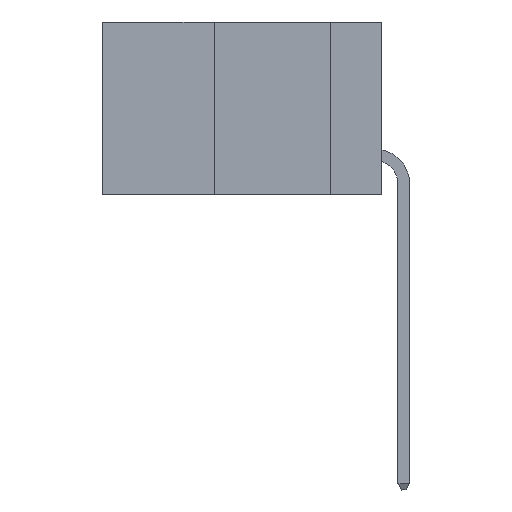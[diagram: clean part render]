
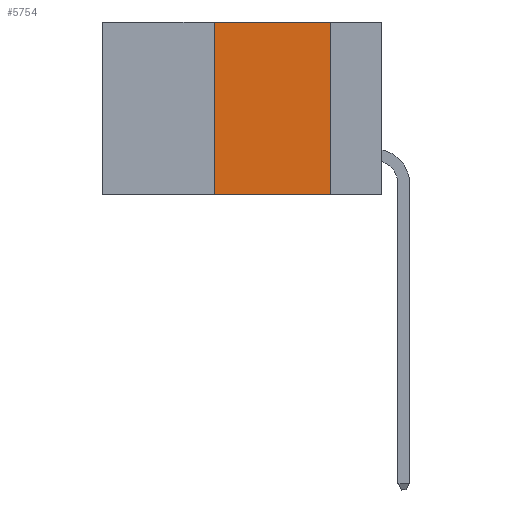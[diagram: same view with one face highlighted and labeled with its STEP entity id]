
A CAD part, left-side view. The second image highlights one B-rep face of the part: STEP entity #5754.
In plain terms, the highlighted planar face has unit normal (-1, 0, 0).
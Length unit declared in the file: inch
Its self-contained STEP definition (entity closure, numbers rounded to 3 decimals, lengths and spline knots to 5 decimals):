
#187 = DIRECTION ( 'NONE',  ( 0., -1., 0. ) ) ;
#1971 = EDGE_CURVE ( 'NONE', #26377, #19439, #18614, .T. ) ;
#2101 = VECTOR ( 'NONE', #187, 39.37008 ) ;
#5494 = EDGE_CURVE ( 'NONE', #26377, #20119, #9552, .T. ) ;
#5586 = CARTESIAN_POINT ( 'NONE',  ( 0., 0.6, 0. ) ) ;
#5754 = ADVANCED_FACE ( 'NONE', ( #17334 ), #20663, .F. ) ;
#5991 = VECTOR ( 'NONE', #29665, 39.37008 ) ;
#6948 = DIRECTION ( 'NONE',  ( 0., 0., -1. ) ) ;
#7227 = VECTOR ( 'NONE', #6948, 39.37008 ) ;
#7928 = CARTESIAN_POINT ( 'NONE',  ( 0., 0.6, 0. ) ) ;
#8650 = EDGE_LOOP ( 'NONE', ( #11639, #40400, #13855, #16289 ) ) ;
#9552 = LINE ( 'NONE', #42589, #5991 ) ;
#10237 = CARTESIAN_POINT ( 'NONE',  ( 0., 0.6, -0.37 ) ) ;
#11639 = ORIENTED_EDGE ( 'NONE', *, *, #19722, .F. ) ;
#13381 = LINE ( 'NONE', #5586, #23776 ) ;
#13855 = ORIENTED_EDGE ( 'NONE', *, *, #5494, .F. ) ;
#16289 = ORIENTED_EDGE ( 'NONE', *, *, #1971, .T. ) ;
#16876 = VERTEX_POINT ( 'NONE', #41990 ) ;
#17334 = FACE_OUTER_BOUND ( 'NONE', #8650, .T. ) ;
#18614 = LINE ( 'NONE', #10237, #2101 ) ;
#19352 = CARTESIAN_POINT ( 'NONE',  ( 0., 0.36, 0. ) ) ;
#19439 = VERTEX_POINT ( 'NONE', #35178 ) ;
#19722 = EDGE_CURVE ( 'NONE', #16876, #19439, #42458, .T. ) ;
#20119 = VERTEX_POINT ( 'NONE', #19352 ) ;
#20663 = PLANE ( 'NONE',  #31442 ) ;
#23776 = VECTOR ( 'NONE', #31764, 39.37008 ) ;
#26377 = VERTEX_POINT ( 'NONE', #39005 ) ;
#26703 = EDGE_CURVE ( 'NONE', #20119, #16876, #13381, .T. ) ;
#27334 = DIRECTION ( 'NONE',  ( 0., 0., -1. ) ) ;
#29665 = DIRECTION ( 'NONE',  ( 0., 0., 1. ) ) ;
#29943 = CARTESIAN_POINT ( 'NONE',  ( 0., 0.11, 0. ) ) ;
#31442 = AXIS2_PLACEMENT_3D ( 'NONE', #7928, #37137, #27334 ) ;
#31764 = DIRECTION ( 'NONE',  ( 0., -1., 0. ) ) ;
#35178 = CARTESIAN_POINT ( 'NONE',  ( 0., 0.11, -0.37 ) ) ;
#37137 = DIRECTION ( 'NONE',  ( 1., 0., 0. ) ) ;
#39005 = CARTESIAN_POINT ( 'NONE',  ( 0., 0.36, -0.37 ) ) ;
#40400 = ORIENTED_EDGE ( 'NONE', *, *, #26703, .F. ) ;
#41990 = CARTESIAN_POINT ( 'NONE',  ( 0., 0.11, 0. ) ) ;
#42458 = LINE ( 'NONE', #29943, #7227 ) ;
#42589 = CARTESIAN_POINT ( 'NONE',  ( 0., 0.36, 0. ) ) ;
